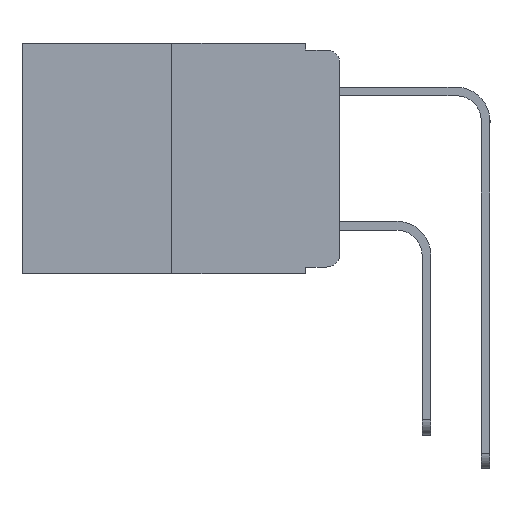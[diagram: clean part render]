
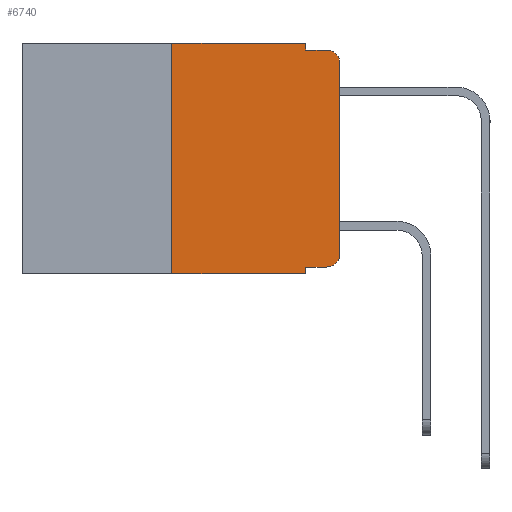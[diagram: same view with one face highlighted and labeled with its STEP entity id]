
A CAD part, left-side view. The second image highlights one B-rep face of the part: STEP entity #6740.
In plain terms, the highlighted planar face has unit normal (-1, 0, 0).
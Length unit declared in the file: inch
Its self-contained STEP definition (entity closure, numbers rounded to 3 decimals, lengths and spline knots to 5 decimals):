
#493 = VERTEX_POINT ( 'NONE', #14894 ) ;
#544 = CARTESIAN_POINT ( 'NONE',  ( 0., 0., -0.313 ) ) ;
#1246 = CIRCLE ( 'NONE', #10460, 0.02 ) ;
#1473 = VERTEX_POINT ( 'NONE', #5247 ) ;
#1876 = DIRECTION ( 'NONE',  ( 0., 0., 1. ) ) ;
#1881 = LINE ( 'NONE', #16754, #10925 ) ;
#2081 = ORIENTED_EDGE ( 'NONE', *, *, #11156, .T. ) ;
#2113 = PLANE ( 'NONE',  #15839 ) ;
#2399 = CARTESIAN_POINT ( 'NONE',  ( 0., 0.473, 0. ) ) ;
#2420 = VERTEX_POINT ( 'NONE', #12373 ) ;
#2569 = CARTESIAN_POINT ( 'NONE',  ( 0., 0.051, 0. ) ) ;
#2759 = EDGE_CURVE ( 'NONE', #493, #13907, #6644, .T. ) ;
#2789 = DIRECTION ( 'NONE',  ( 0., 0., 1. ) ) ;
#3602 = DIRECTION ( 'NONE',  ( 0., 0., -1. ) ) ;
#3651 = EDGE_CURVE ( 'NONE', #1473, #13907, #11757, .T. ) ;
#3687 = LINE ( 'NONE', #13237, #10291 ) ;
#3711 = CARTESIAN_POINT ( 'NONE',  ( 0., 0.051, -0.333 ) ) ;
#3982 = EDGE_CURVE ( 'NONE', #5822, #1473, #8026, .T. ) ;
#4148 = ORIENTED_EDGE ( 'NONE', *, *, #4599, .T. ) ;
#4511 = EDGE_CURVE ( 'NONE', #4980, #14818, #10342, .T. ) ;
#4599 = EDGE_CURVE ( 'NONE', #8944, #14818, #1881, .T. ) ;
#4980 = VERTEX_POINT ( 'NONE', #7949 ) ;
#5247 = CARTESIAN_POINT ( 'NONE',  ( 0., 0.051, -0.01 ) ) ;
#5604 = LINE ( 'NONE', #2399, #8655 ) ;
#5822 = VERTEX_POINT ( 'NONE', #2569 ) ;
#5986 = EDGE_CURVE ( 'NONE', #8944, #2420, #3687, .T. ) ;
#6503 = LINE ( 'NONE', #3711, #9095 ) ;
#6543 = ORIENTED_EDGE ( 'NONE', *, *, #3982, .F. ) ;
#6637 = CARTESIAN_POINT ( 'NONE',  ( 0., 0.02, -0.313 ) ) ;
#6644 = CIRCLE ( 'NONE', #16367, 0.02 ) ;
#6740 = ADVANCED_FACE ( 'NONE', ( #16195 ), #2113, .F. ) ;
#6919 = CARTESIAN_POINT ( 'NONE',  ( 0., 0.25, -0.343 ) ) ;
#7258 = EDGE_CURVE ( 'NONE', #4980, #14903, #6503, .T. ) ;
#7506 = DIRECTION ( 'NONE',  ( 0., 0., -1. ) ) ;
#7695 = CARTESIAN_POINT ( 'NONE',  ( 0., 0.473, 0. ) ) ;
#7739 = EDGE_CURVE ( 'NONE', #10883, #493, #14978, .T. ) ;
#7904 = DIRECTION ( 'NONE',  ( 0., 0., -1. ) ) ;
#7937 = DIRECTION ( 'NONE',  ( 0., 0., -1. ) ) ;
#7949 = CARTESIAN_POINT ( 'NONE',  ( 0., 0.051, -0.333 ) ) ;
#8026 = LINE ( 'NONE', #13730, #13480 ) ;
#8171 = ORIENTED_EDGE ( 'NONE', *, *, #4511, .F. ) ;
#8655 = VECTOR ( 'NONE', #10433, 39.37008 ) ;
#8680 = VECTOR ( 'NONE', #1876, 39.37008 ) ;
#8732 = ORIENTED_EDGE ( 'NONE', *, *, #7739, .T. ) ;
#8780 = EDGE_CURVE ( 'NONE', #2420, #5822, #5604, .T. ) ;
#8944 = VERTEX_POINT ( 'NONE', #6919 ) ;
#9095 = VECTOR ( 'NONE', #15308, 39.37008 ) ;
#9119 = EDGE_LOOP ( 'NONE', ( #8732, #15428, #16237, #6543, #13623, #10697, #4148, #8171, #15243, #2081 ) ) ;
#9977 = CARTESIAN_POINT ( 'NONE',  ( 0., 0., 0. ) ) ;
#10291 = VECTOR ( 'NONE', #2789, 39.37008 ) ;
#10342 = LINE ( 'NONE', #16490, #12867 ) ;
#10433 = DIRECTION ( 'NONE',  ( 0., -1., 0. ) ) ;
#10450 = CARTESIAN_POINT ( 'NONE',  ( 0., 0.02, -0.333 ) ) ;
#10460 = AXIS2_PLACEMENT_3D ( 'NONE', #6637, #15468, #7937 ) ;
#10469 = DIRECTION ( 'NONE',  ( 0., -1., 0. ) ) ;
#10697 = ORIENTED_EDGE ( 'NONE', *, *, #5986, .F. ) ;
#10883 = VERTEX_POINT ( 'NONE', #544 ) ;
#10925 = VECTOR ( 'NONE', #10469, 39.37008 ) ;
#11156 = EDGE_CURVE ( 'NONE', #14903, #10883, #1246, .T. ) ;
#11365 = VECTOR ( 'NONE', #16537, 39.37008 ) ;
#11473 = DIRECTION ( 'NONE',  ( 1., 0., 0. ) ) ;
#11532 = CARTESIAN_POINT ( 'NONE',  ( 0., 0.02, -0.01 ) ) ;
#11757 = LINE ( 'NONE', #15924, #11365 ) ;
#12373 = CARTESIAN_POINT ( 'NONE',  ( 0., 0.25, 0. ) ) ;
#12867 = VECTOR ( 'NONE', #15229, 39.37008 ) ;
#13237 = CARTESIAN_POINT ( 'NONE',  ( 0., 0.25, 0. ) ) ;
#13480 = VECTOR ( 'NONE', #7506, 39.37008 ) ;
#13623 = ORIENTED_EDGE ( 'NONE', *, *, #8780, .F. ) ;
#13730 = CARTESIAN_POINT ( 'NONE',  ( 0., 0.051, 0. ) ) ;
#13907 = VERTEX_POINT ( 'NONE', #11532 ) ;
#14818 = VERTEX_POINT ( 'NONE', #15373 ) ;
#14894 = CARTESIAN_POINT ( 'NONE',  ( 0., 0., -0.03 ) ) ;
#14903 = VERTEX_POINT ( 'NONE', #10450 ) ;
#14978 = LINE ( 'NONE', #9977, #8680 ) ;
#15229 = DIRECTION ( 'NONE',  ( 0., 0., -1. ) ) ;
#15243 = ORIENTED_EDGE ( 'NONE', *, *, #7258, .T. ) ;
#15308 = DIRECTION ( 'NONE',  ( 0., -1., 0. ) ) ;
#15373 = CARTESIAN_POINT ( 'NONE',  ( 0., 0.051, -0.343 ) ) ;
#15428 = ORIENTED_EDGE ( 'NONE', *, *, #2759, .T. ) ;
#15468 = DIRECTION ( 'NONE',  ( -1., 0., 0. ) ) ;
#15625 = DIRECTION ( 'NONE',  ( -1., 0., 0. ) ) ;
#15681 = CARTESIAN_POINT ( 'NONE',  ( 0., 0.02, -0.03 ) ) ;
#15839 = AXIS2_PLACEMENT_3D ( 'NONE', #7695, #11473, #3602 ) ;
#15924 = CARTESIAN_POINT ( 'NONE',  ( 0., 0.051, -0.01 ) ) ;
#16195 = FACE_OUTER_BOUND ( 'NONE', #9119, .T. ) ;
#16237 = ORIENTED_EDGE ( 'NONE', *, *, #3651, .F. ) ;
#16367 = AXIS2_PLACEMENT_3D ( 'NONE', #15681, #15625, #7904 ) ;
#16490 = CARTESIAN_POINT ( 'NONE',  ( 0., 0.051, 0. ) ) ;
#16537 = DIRECTION ( 'NONE',  ( 0., -1., 0. ) ) ;
#16754 = CARTESIAN_POINT ( 'NONE',  ( 0., 0.473, -0.343 ) ) ;
